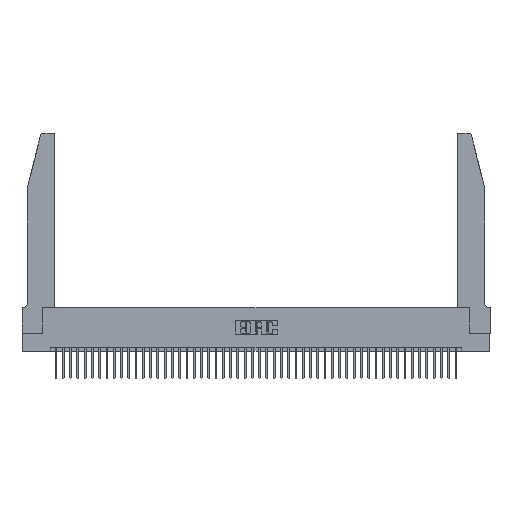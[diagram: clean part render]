
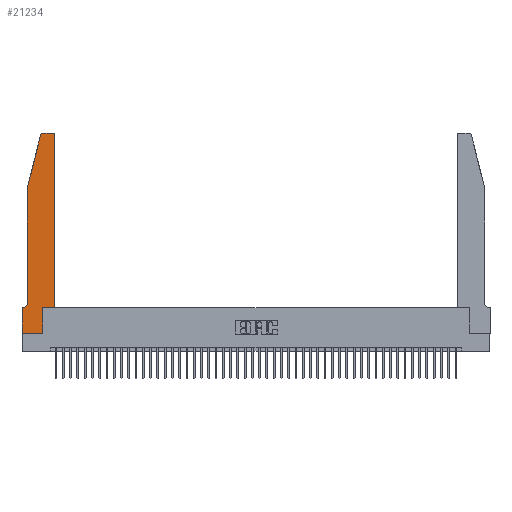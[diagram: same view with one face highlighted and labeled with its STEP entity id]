
A CAD part, top view. The second image highlights one B-rep face of the part: STEP entity #21234.
In plain terms, the highlighted planar face has unit normal (0, 0, 1).
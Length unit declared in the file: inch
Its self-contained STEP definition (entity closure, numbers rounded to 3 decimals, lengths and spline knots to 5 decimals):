
#117 = EDGE_CURVE ( 'NONE', #18294, #10794, #10117, .T. ) ;
#1149 = DIRECTION ( 'NONE',  ( -0.239, -0.971, 0. ) ) ;
#1435 = EDGE_CURVE ( 'NONE', #16065, #23384, #2074, .T. ) ;
#1485 = LINE ( 'NONE', #6613, #21312 ) ;
#1500 = DIRECTION ( 'NONE',  ( 0., 0., -1. ) ) ;
#1546 = CARTESIAN_POINT ( 'NONE',  ( 0.4205, 2.72, 0.37 ) ) ;
#1647 = VECTOR ( 'NONE', #1149, 39.37008 ) ;
#1665 = DIRECTION ( 'NONE',  ( 1., 0., 0. ) ) ;
#2074 = CIRCLE ( 'NONE', #12737, 0.03 ) ;
#3411 = VECTOR ( 'NONE', #37299, 39.37008 ) ;
#3502 = CARTESIAN_POINT ( 'NONE',  ( 0.4505, 0.35, 0.37 ) ) ;
#3545 = ORIENTED_EDGE ( 'NONE', *, *, #9262, .T. ) ;
#3980 = CARTESIAN_POINT ( 'NONE',  ( 0.2865, 0., 0.37 ) ) ;
#4130 = CARTESIAN_POINT ( 'NONE',  ( 0.2865, 0.35, 0.37 ) ) ;
#4492 = LINE ( 'NONE', #41139, #35083 ) ;
#4957 = VECTOR ( 'NONE', #33716, 39.37008 ) ;
#5557 = VECTOR ( 'NONE', #30602, 39.37008 ) ;
#5620 = ORIENTED_EDGE ( 'NONE', *, *, #117, .T. ) ;
#5796 = CARTESIAN_POINT ( 'NONE',  ( 0.4505, 2.72, 0.37 ) ) ;
#6291 = VECTOR ( 'NONE', #23704, 39.37008 ) ;
#6613 = CARTESIAN_POINT ( 'NONE',  ( 0.2605, 2.75, 0.37 ) ) ;
#6861 = ORIENTED_EDGE ( 'NONE', *, *, #44121, .T. ) ;
#7050 = FACE_OUTER_BOUND ( 'NONE', #13156, .T. ) ;
#7822 = DIRECTION ( 'NONE',  ( -1., 0., 0. ) ) ;
#8558 = CIRCLE ( 'NONE', #26406, 0.03 ) ;
#8749 = CIRCLE ( 'NONE', #38026, 0.07 ) ;
#9262 = EDGE_CURVE ( 'NONE', #10794, #12257, #8749, .T. ) ;
#9945 = ORIENTED_EDGE ( 'NONE', *, *, #17554, .T. ) ;
#10117 = LINE ( 'NONE', #29633, #5557 ) ;
#10610 = EDGE_CURVE ( 'NONE', #12823, #26831, #11856, .T. ) ;
#10794 = VERTEX_POINT ( 'NONE', #16325 ) ;
#11206 = VECTOR ( 'NONE', #7822, 39.37008 ) ;
#11315 = LINE ( 'NONE', #22830, #1647 ) ;
#11856 = LINE ( 'NONE', #42890, #25389 ) ;
#12257 = VERTEX_POINT ( 'NONE', #21691 ) ;
#12737 = AXIS2_PLACEMENT_3D ( 'NONE', #45269, #23574, #16472 ) ;
#12823 = VERTEX_POINT ( 'NONE', #13540 ) ;
#13156 = EDGE_LOOP ( 'NONE', ( #31756, #34263, #25533, #5620, #3545, #6861, #24282, #19813, #22096, #9945, #13979, #19216 ) ) ;
#13540 = CARTESIAN_POINT ( 'NONE',  ( 0., 0.35, 0.37 ) ) ;
#13979 = ORIENTED_EDGE ( 'NONE', *, *, #18750, .T. ) ;
#14191 = LINE ( 'NONE', #44145, #3411 ) ;
#14382 = DIRECTION ( 'NONE',  ( 0., -1., 0. ) ) ;
#14977 = VERTEX_POINT ( 'NONE', #5796 ) ;
#15968 = DIRECTION ( 'NONE',  ( 1., 0., 0. ) ) ;
#16041 = EDGE_CURVE ( 'NONE', #14977, #37599, #8558, .T. ) ;
#16065 = VERTEX_POINT ( 'NONE', #41250 ) ;
#16325 = CARTESIAN_POINT ( 'NONE',  ( 0.0755, 0.42, 0.37 ) ) ;
#16472 = DIRECTION ( 'NONE',  ( 1., 0., 0. ) ) ;
#16665 = EDGE_CURVE ( 'NONE', #23384, #18294, #11315, .T. ) ;
#17376 = LINE ( 'NONE', #28353, #4957 ) ;
#17554 = EDGE_CURVE ( 'NONE', #40262, #19169, #4492, .T. ) ;
#17936 = CARTESIAN_POINT ( 'NONE',  ( 0., 0., 0.37 ) ) ;
#18294 = VERTEX_POINT ( 'NONE', #28356 ) ;
#18750 = EDGE_CURVE ( 'NONE', #19169, #14977, #17376, .T. ) ;
#19169 = VERTEX_POINT ( 'NONE', #3502 ) ;
#19216 = ORIENTED_EDGE ( 'NONE', *, *, #16041, .T. ) ;
#19813 = ORIENTED_EDGE ( 'NONE', *, *, #36479, .T. ) ;
#19885 = DIRECTION ( 'NONE',  ( -1., 0., 0. ) ) ;
#21163 = CARTESIAN_POINT ( 'NONE',  ( 0.25487, 2.72718, 0.37 ) ) ;
#21234 = ADVANCED_FACE ( 'NONE', ( #7050 ), #34097, .T. ) ;
#21312 = VECTOR ( 'NONE', #39140, 39.37008 ) ;
#21691 = CARTESIAN_POINT ( 'NONE',  ( 0.0055, 0.35, 0.37 ) ) ;
#22096 = ORIENTED_EDGE ( 'NONE', *, *, #23247, .T. ) ;
#22830 = CARTESIAN_POINT ( 'NONE',  ( 0.0755, 2., 0.37 ) ) ;
#23025 = LINE ( 'NONE', #44179, #11206 ) ;
#23247 = EDGE_CURVE ( 'NONE', #40224, #40262, #33404, .T. ) ;
#23328 = DIRECTION ( 'NONE',  ( 0., 0., 1. ) ) ;
#23384 = VERTEX_POINT ( 'NONE', #21163 ) ;
#23574 = DIRECTION ( 'NONE',  ( 0., 0., 1. ) ) ;
#23704 = DIRECTION ( 'NONE',  ( 0., 1., 0. ) ) ;
#23865 = EDGE_CURVE ( 'NONE', #37599, #16065, #1485, .T. ) ;
#24282 = ORIENTED_EDGE ( 'NONE', *, *, #10610, .T. ) ;
#25068 = CARTESIAN_POINT ( 'NONE',  ( 0.4205, 2.75, 0.37 ) ) ;
#25389 = VECTOR ( 'NONE', #14382, 39.37008 ) ;
#25533 = ORIENTED_EDGE ( 'NONE', *, *, #16665, .T. ) ;
#26406 = AXIS2_PLACEMENT_3D ( 'NONE', #1546, #33988, #15968 ) ;
#26831 = VERTEX_POINT ( 'NONE', #17936 ) ;
#28353 = CARTESIAN_POINT ( 'NONE',  ( 0.4505, 0.35, 0.37 ) ) ;
#28356 = CARTESIAN_POINT ( 'NONE',  ( 0.0755, 2., 0.37 ) ) ;
#29633 = CARTESIAN_POINT ( 'NONE',  ( 0.0755, 2., 0.37 ) ) ;
#30602 = DIRECTION ( 'NONE',  ( 0., -1., 0. ) ) ;
#31756 = ORIENTED_EDGE ( 'NONE', *, *, #23865, .T. ) ;
#33404 = LINE ( 'NONE', #45242, #6291 ) ;
#33598 = AXIS2_PLACEMENT_3D ( 'NONE', #41355, #23328, #1665 ) ;
#33716 = DIRECTION ( 'NONE',  ( 0., 1., 0. ) ) ;
#33988 = DIRECTION ( 'NONE',  ( 0., 0., 1. ) ) ;
#34097 = PLANE ( 'NONE',  #33598 ) ;
#34263 = ORIENTED_EDGE ( 'NONE', *, *, #1435, .T. ) ;
#35083 = VECTOR ( 'NONE', #37179, 39.37008 ) ;
#36479 = EDGE_CURVE ( 'NONE', #26831, #40224, #14191, .T. ) ;
#37179 = DIRECTION ( 'NONE',  ( 1., 0., 0. ) ) ;
#37299 = DIRECTION ( 'NONE',  ( 1., 0., 0. ) ) ;
#37599 = VERTEX_POINT ( 'NONE', #25068 ) ;
#37884 = CARTESIAN_POINT ( 'NONE',  ( 0.0055, 0.42, 0.37 ) ) ;
#38026 = AXIS2_PLACEMENT_3D ( 'NONE', #37884, #1500, #19885 ) ;
#39140 = DIRECTION ( 'NONE',  ( -1., 0., 0. ) ) ;
#40224 = VERTEX_POINT ( 'NONE', #3980 ) ;
#40262 = VERTEX_POINT ( 'NONE', #4130 ) ;
#41139 = CARTESIAN_POINT ( 'NONE',  ( 0.4505, 0.35, 0.37 ) ) ;
#41250 = CARTESIAN_POINT ( 'NONE',  ( 0.284, 2.75, 0.37 ) ) ;
#41355 = CARTESIAN_POINT ( 'NONE',  ( 0., 0.35, 0.37 ) ) ;
#42890 = CARTESIAN_POINT ( 'NONE',  ( 0., 0., 0.37 ) ) ;
#44121 = EDGE_CURVE ( 'NONE', #12257, #12823, #23025, .T. ) ;
#44145 = CARTESIAN_POINT ( 'NONE',  ( 0., 0., 0.37 ) ) ;
#44179 = CARTESIAN_POINT ( 'NONE',  ( 0.0755, 0.35, 0.37 ) ) ;
#45242 = CARTESIAN_POINT ( 'NONE',  ( 0.2865, 0.35, 0.37 ) ) ;
#45269 = CARTESIAN_POINT ( 'NONE',  ( 0.284, 2.72, 0.37 ) ) ;
